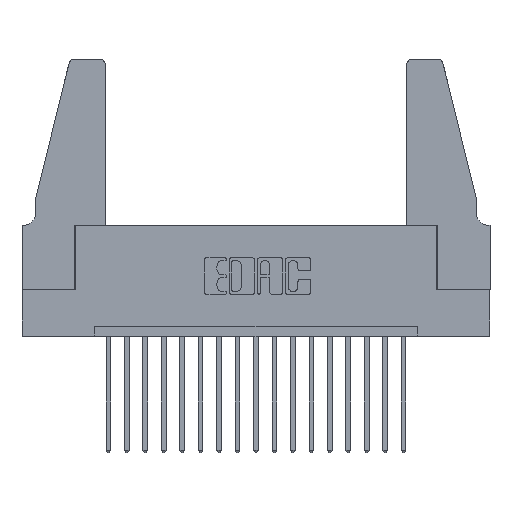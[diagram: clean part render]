
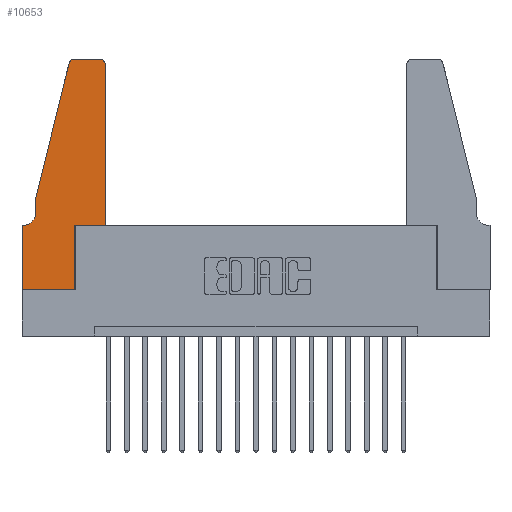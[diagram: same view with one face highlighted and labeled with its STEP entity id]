
A CAD part, top view. The second image highlights one B-rep face of the part: STEP entity #10653.
In plain terms, the highlighted planar face has unit normal (0, 0, 1).
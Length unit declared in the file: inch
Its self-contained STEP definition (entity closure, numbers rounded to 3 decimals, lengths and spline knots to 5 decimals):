
#136 = VERTEX_POINT ( 'NONE', #14775 ) ;
#284 = LINE ( 'NONE', #13048, #5139 ) ;
#429 = DIRECTION ( 'NONE',  ( -1., 0., 0. ) ) ;
#886 = VECTOR ( 'NONE', #2533, 39.37008 ) ;
#1084 = ORIENTED_EDGE ( 'NONE', *, *, #16691, .T. ) ;
#1282 = ORIENTED_EDGE ( 'NONE', *, *, #6268, .T. ) ;
#1302 = DIRECTION ( 'NONE',  ( 1., 0., 0. ) ) ;
#1527 = VERTEX_POINT ( 'NONE', #6563 ) ;
#1545 = VERTEX_POINT ( 'NONE', #3777 ) ;
#2233 = LINE ( 'NONE', #9224, #16667 ) ;
#2533 = DIRECTION ( 'NONE',  ( 0., 1., 0. ) ) ;
#3042 = CARTESIAN_POINT ( 'NONE',  ( 0.2865, 0.35, 0.37 ) ) ;
#3342 = VERTEX_POINT ( 'NONE', #3042 ) ;
#3434 = CARTESIAN_POINT ( 'NONE',  ( 0., 0., 0.37 ) ) ;
#3450 = VECTOR ( 'NONE', #16255, 39.37008 ) ;
#3484 = CARTESIAN_POINT ( 'NONE',  ( 0.0755, 0.5, 0.37 ) ) ;
#3497 = EDGE_CURVE ( 'NONE', #6250, #1545, #5488, .T. ) ;
#3552 = EDGE_CURVE ( 'NONE', #3342, #13396, #17458, .T. ) ;
#3553 = CARTESIAN_POINT ( 'NONE',  ( 0.4505, 1.22, 0.37 ) ) ;
#3777 = CARTESIAN_POINT ( 'NONE',  ( 0.284, 1.25, 0.37 ) ) ;
#3926 = EDGE_LOOP ( 'NONE', ( #4789, #13672, #1084, #15503, #17081, #13366, #14764, #1282, #4410, #6047, #17341, #13854 ) ) ;
#3971 = LINE ( 'NONE', #12860, #10364 ) ;
#4184 = CARTESIAN_POINT ( 'NONE',  ( 0.4205, 1.22, 0.37 ) ) ;
#4237 = CIRCLE ( 'NONE', #17412, 0.07 ) ;
#4410 = ORIENTED_EDGE ( 'NONE', *, *, #8068, .T. ) ;
#4789 = ORIENTED_EDGE ( 'NONE', *, *, #3497, .T. ) ;
#4805 = AXIS2_PLACEMENT_3D ( 'NONE', #4939, #10329, #7553 ) ;
#4939 = CARTESIAN_POINT ( 'NONE',  ( 0.284, 1.22, 0.37 ) ) ;
#4945 = DIRECTION ( 'NONE',  ( -1., 0., 0. ) ) ;
#5077 = DIRECTION ( 'NONE',  ( -1., 0., 0. ) ) ;
#5139 = VECTOR ( 'NONE', #14494, 39.37008 ) ;
#5320 = CIRCLE ( 'NONE', #10975, 0.03 ) ;
#5488 = LINE ( 'NONE', #7870, #10785 ) ;
#5649 = CARTESIAN_POINT ( 'NONE',  ( 0., 0., 0.37 ) ) ;
#5661 = DIRECTION ( 'NONE',  ( 1., 0., 0. ) ) ;
#6047 = ORIENTED_EDGE ( 'NONE', *, *, #3552, .T. ) ;
#6059 = VECTOR ( 'NONE', #1302, 39.37008 ) ;
#6250 = VERTEX_POINT ( 'NONE', #6955 ) ;
#6268 = EDGE_CURVE ( 'NONE', #11488, #136, #10250, .T. ) ;
#6563 = CARTESIAN_POINT ( 'NONE',  ( 0., 0.35, 0.37 ) ) ;
#6756 = CARTESIAN_POINT ( 'NONE',  ( 0., 0.35, 0.37 ) ) ;
#6779 = EDGE_CURVE ( 'NONE', #1545, #18078, #17338, .T. ) ;
#6955 = CARTESIAN_POINT ( 'NONE',  ( 0.4205, 1.25, 0.37 ) ) ;
#7553 = DIRECTION ( 'NONE',  ( 1., 0., 0. ) ) ;
#7616 = EDGE_CURVE ( 'NONE', #11324, #17422, #4237, .T. ) ;
#7870 = CARTESIAN_POINT ( 'NONE',  ( 0.2605, 1.25, 0.37 ) ) ;
#7982 = CARTESIAN_POINT ( 'NONE',  ( 0.0755, 0.5, 0.37 ) ) ;
#8068 = EDGE_CURVE ( 'NONE', #136, #3342, #14196, .T. ) ;
#8100 = CARTESIAN_POINT ( 'NONE',  ( 0.0055, 0.42, 0.37 ) ) ;
#8385 = EDGE_CURVE ( 'NONE', #8848, #6250, #5320, .T. ) ;
#8544 = DIRECTION ( 'NONE',  ( 1., 0., 0. ) ) ;
#8848 = VERTEX_POINT ( 'NONE', #3553 ) ;
#8856 = EDGE_CURVE ( 'NONE', #1527, #11488, #2233, .T. ) ;
#9016 = VECTOR ( 'NONE', #18141, 39.37008 ) ;
#9158 = DIRECTION ( 'NONE',  ( -0.239, -0.971, 0. ) ) ;
#9224 = CARTESIAN_POINT ( 'NONE',  ( 0., 0., 0.37 ) ) ;
#9524 = VECTOR ( 'NONE', #9158, 39.37008 ) ;
#9703 = CARTESIAN_POINT ( 'NONE',  ( 0.4505, 0.35, 0.37 ) ) ;
#9882 = VERTEX_POINT ( 'NONE', #15886 ) ;
#10166 = FACE_OUTER_BOUND ( 'NONE', #3926, .T. ) ;
#10250 = LINE ( 'NONE', #5649, #6059 ) ;
#10329 = DIRECTION ( 'NONE',  ( 0., 0., 1. ) ) ;
#10364 = VECTOR ( 'NONE', #429, 39.37008 ) ;
#10653 = ADVANCED_FACE ( 'NONE', ( #10166 ), #15236, .T. ) ;
#10691 = EDGE_CURVE ( 'NONE', #17422, #1527, #3971, .T. ) ;
#10785 = VECTOR ( 'NONE', #5077, 39.37008 ) ;
#10975 = AXIS2_PLACEMENT_3D ( 'NONE', #4184, #12697, #5661 ) ;
#11273 = CARTESIAN_POINT ( 'NONE',  ( 0.2865, 0.35, 0.37 ) ) ;
#11324 = VERTEX_POINT ( 'NONE', #15204 ) ;
#11434 = CARTESIAN_POINT ( 'NONE',  ( 0.0055, 0.35, 0.37 ) ) ;
#11488 = VERTEX_POINT ( 'NONE', #3434 ) ;
#12697 = DIRECTION ( 'NONE',  ( 0., 0., 1. ) ) ;
#12860 = CARTESIAN_POINT ( 'NONE',  ( 0.0755, 0.35, 0.37 ) ) ;
#13048 = CARTESIAN_POINT ( 'NONE',  ( 0.4505, 0.35, 0.37 ) ) ;
#13085 = EDGE_CURVE ( 'NONE', #9882, #11324, #17867, .T. ) ;
#13366 = ORIENTED_EDGE ( 'NONE', *, *, #10691, .T. ) ;
#13396 = VERTEX_POINT ( 'NONE', #14083 ) ;
#13416 = AXIS2_PLACEMENT_3D ( 'NONE', #6756, #18077, #8544 ) ;
#13482 = CARTESIAN_POINT ( 'NONE',  ( 0.25487, 1.22718, 0.37 ) ) ;
#13672 = ORIENTED_EDGE ( 'NONE', *, *, #6779, .T. ) ;
#13854 = ORIENTED_EDGE ( 'NONE', *, *, #8385, .T. ) ;
#14083 = CARTESIAN_POINT ( 'NONE',  ( 0.4505, 0.35, 0.37 ) ) ;
#14196 = LINE ( 'NONE', #11273, #886 ) ;
#14494 = DIRECTION ( 'NONE',  ( 0., 1., 0. ) ) ;
#14647 = LINE ( 'NONE', #3484, #9524 ) ;
#14764 = ORIENTED_EDGE ( 'NONE', *, *, #8856, .T. ) ;
#14775 = CARTESIAN_POINT ( 'NONE',  ( 0.2865, 0., 0.37 ) ) ;
#14803 = DIRECTION ( 'NONE',  ( 0., 0., -1. ) ) ;
#15204 = CARTESIAN_POINT ( 'NONE',  ( 0.0755, 0.42, 0.37 ) ) ;
#15236 = PLANE ( 'NONE',  #13416 ) ;
#15503 = ORIENTED_EDGE ( 'NONE', *, *, #13085, .T. ) ;
#15872 = EDGE_CURVE ( 'NONE', #13396, #8848, #284, .T. ) ;
#15886 = CARTESIAN_POINT ( 'NONE',  ( 0.0755, 0.5, 0.37 ) ) ;
#16255 = DIRECTION ( 'NONE',  ( 0., -1., 0. ) ) ;
#16667 = VECTOR ( 'NONE', #17612, 39.37008 ) ;
#16691 = EDGE_CURVE ( 'NONE', #18078, #9882, #14647, .T. ) ;
#17081 = ORIENTED_EDGE ( 'NONE', *, *, #7616, .T. ) ;
#17338 = CIRCLE ( 'NONE', #4805, 0.03 ) ;
#17341 = ORIENTED_EDGE ( 'NONE', *, *, #15872, .T. ) ;
#17412 = AXIS2_PLACEMENT_3D ( 'NONE', #8100, #14803, #4945 ) ;
#17422 = VERTEX_POINT ( 'NONE', #11434 ) ;
#17458 = LINE ( 'NONE', #9703, #9016 ) ;
#17612 = DIRECTION ( 'NONE',  ( 0., -1., 0. ) ) ;
#17867 = LINE ( 'NONE', #7982, #3450 ) ;
#18077 = DIRECTION ( 'NONE',  ( 0., 0., 1. ) ) ;
#18078 = VERTEX_POINT ( 'NONE', #13482 ) ;
#18141 = DIRECTION ( 'NONE',  ( 1., 0., 0. ) ) ;
